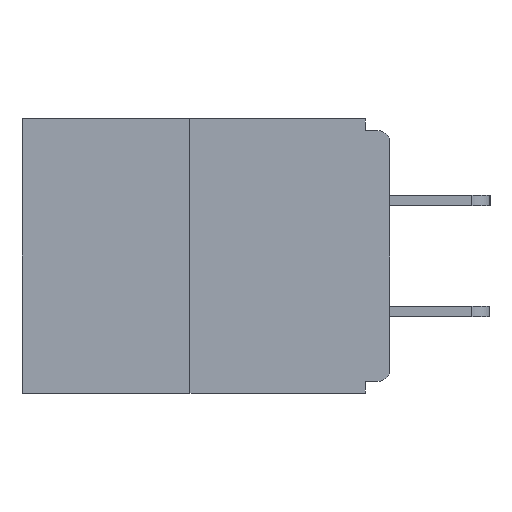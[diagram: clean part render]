
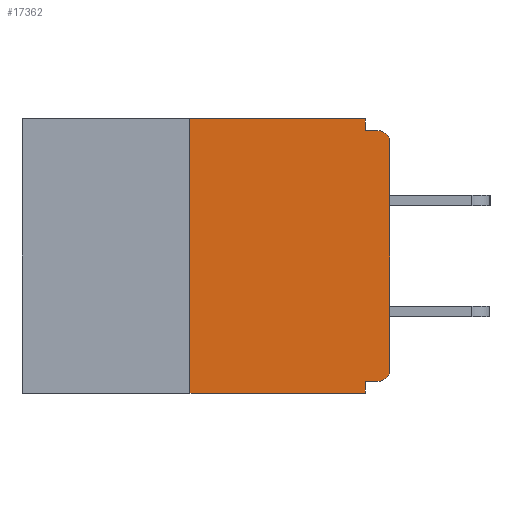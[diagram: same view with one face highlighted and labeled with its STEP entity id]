
A CAD part, left-side view. The second image highlights one B-rep face of the part: STEP entity #17362.
In plain terms, the highlighted planar face has unit normal (-1, 0, 0).
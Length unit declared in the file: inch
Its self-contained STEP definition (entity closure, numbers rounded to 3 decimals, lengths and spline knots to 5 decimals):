
#633 = DIRECTION ( 'NONE',  ( -1., 0., 0. ) ) ;
#658 = LINE ( 'NONE', #7552, #6384 ) ;
#696 = ORIENTED_EDGE ( 'NONE', *, *, #22008, .F. ) ;
#698 = CARTESIAN_POINT ( 'NONE',  ( 0., 0.031, -0.343 ) ) ;
#746 = CARTESIAN_POINT ( 'NONE',  ( 0., 0.031, 0. ) ) ;
#1198 = VECTOR ( 'NONE', #19007, 39.37008 ) ;
#1245 = CIRCLE ( 'NONE', #4268, 0.015 ) ;
#1702 = CARTESIAN_POINT ( 'NONE',  ( 0., 0.46, -0.343 ) ) ;
#2007 = VECTOR ( 'NONE', #16914, 39.37008 ) ;
#2011 = ORIENTED_EDGE ( 'NONE', *, *, #13582, .F. ) ;
#2282 = EDGE_CURVE ( 'NONE', #7714, #10179, #658, .T. ) ;
#2679 = PLANE ( 'NONE',  #21142 ) ;
#2697 = VERTEX_POINT ( 'NONE', #16904 ) ;
#2753 = EDGE_CURVE ( 'NONE', #10179, #21299, #7271, .T. ) ;
#2975 = CARTESIAN_POINT ( 'NONE',  ( 0., 0., -0.313 ) ) ;
#3188 = CARTESIAN_POINT ( 'NONE',  ( 0., 0.25, 0. ) ) ;
#4268 = AXIS2_PLACEMENT_3D ( 'NONE', #5613, #16413, #18456 ) ;
#4496 = LINE ( 'NONE', #698, #1198 ) ;
#4762 = ORIENTED_EDGE ( 'NONE', *, *, #13881, .T. ) ;
#4852 = ORIENTED_EDGE ( 'NONE', *, *, #16057, .F. ) ;
#5162 = CARTESIAN_POINT ( 'NONE',  ( 0., 0., -0.015 ) ) ;
#5386 = LINE ( 'NONE', #5162, #18011 ) ;
#5613 = CARTESIAN_POINT ( 'NONE',  ( 0., 0.015, -0.313 ) ) ;
#5687 = CARTESIAN_POINT ( 'NONE',  ( 0., 0.25, 0. ) ) ;
#5970 = DIRECTION ( 'NONE',  ( 0., 0., -1. ) ) ;
#5994 = EDGE_LOOP ( 'NONE', ( #7019, #18274, #4762, #4852, #2011, #18124, #6277, #15535, #7872, #696 ) ) ;
#6277 = ORIENTED_EDGE ( 'NONE', *, *, #2282, .T. ) ;
#6374 = CARTESIAN_POINT ( 'NONE',  ( 0., 0.015, -0.328 ) ) ;
#6384 = VECTOR ( 'NONE', #18962, 39.37008 ) ;
#6940 = LINE ( 'NONE', #1702, #16783 ) ;
#7019 = ORIENTED_EDGE ( 'NONE', *, *, #7269, .F. ) ;
#7269 = EDGE_CURVE ( 'NONE', #18222, #12796, #14925, .T. ) ;
#7271 = CIRCLE ( 'NONE', #18394, 0.015 ) ;
#7540 = CARTESIAN_POINT ( 'NONE',  ( 0., 0., -0.328 ) ) ;
#7552 = CARTESIAN_POINT ( 'NONE',  ( 0., 0., 0. ) ) ;
#7714 = VERTEX_POINT ( 'NONE', #2975 ) ;
#7872 = ORIENTED_EDGE ( 'NONE', *, *, #20592, .F. ) ;
#8287 = CARTESIAN_POINT ( 'NONE',  ( 0., 0.46, 0. ) ) ;
#8774 = VECTOR ( 'NONE', #14571, 39.37008 ) ;
#9025 = CARTESIAN_POINT ( 'NONE',  ( 0., 0.46, 0. ) ) ;
#9357 = DIRECTION ( 'NONE',  ( 0., -1., 0. ) ) ;
#9393 = EDGE_CURVE ( 'NONE', #10746, #7714, #1245, .T. ) ;
#9884 = VECTOR ( 'NONE', #11315, 39.37008 ) ;
#10179 = VERTEX_POINT ( 'NONE', #17896 ) ;
#10746 = VERTEX_POINT ( 'NONE', #6374 ) ;
#11239 = CARTESIAN_POINT ( 'NONE',  ( 0., 0.031, -0.015 ) ) ;
#11315 = DIRECTION ( 'NONE',  ( 0., 1., 0. ) ) ;
#11369 = DIRECTION ( 'NONE',  ( 0., 0., 1. ) ) ;
#11543 = LINE ( 'NONE', #746, #2007 ) ;
#11707 = DIRECTION ( 'NONE',  ( 1., 0., 0. ) ) ;
#12796 = VERTEX_POINT ( 'NONE', #22966 ) ;
#13266 = VERTEX_POINT ( 'NONE', #19332 ) ;
#13582 = EDGE_CURVE ( 'NONE', #10746, #2697, #16565, .T. ) ;
#13850 = VECTOR ( 'NONE', #11369, 39.37008 ) ;
#13881 = EDGE_CURVE ( 'NONE', #16589, #13266, #6940, .T. ) ;
#14298 = DIRECTION ( 'NONE',  ( 0., -1., 0. ) ) ;
#14571 = DIRECTION ( 'NONE',  ( 0., -1., 0. ) ) ;
#14925 = LINE ( 'NONE', #9025, #8774 ) ;
#15535 = ORIENTED_EDGE ( 'NONE', *, *, #2753, .T. ) ;
#15632 = DIRECTION ( 'NONE',  ( 0., 0., -1. ) ) ;
#16057 = EDGE_CURVE ( 'NONE', #2697, #13266, #4496, .T. ) ;
#16413 = DIRECTION ( 'NONE',  ( -1., 0., 0. ) ) ;
#16565 = LINE ( 'NONE', #7540, #9884 ) ;
#16589 = VERTEX_POINT ( 'NONE', #17599 ) ;
#16783 = VECTOR ( 'NONE', #14298, 39.37008 ) ;
#16847 = EDGE_CURVE ( 'NONE', #16589, #18222, #22118, .T. ) ;
#16904 = CARTESIAN_POINT ( 'NONE',  ( 0., 0.031, -0.328 ) ) ;
#16914 = DIRECTION ( 'NONE',  ( 0., 0., -1. ) ) ;
#17362 = ADVANCED_FACE ( 'NONE', ( #23078 ), #2679, .F. ) ;
#17599 = CARTESIAN_POINT ( 'NONE',  ( 0., 0.25, -0.343 ) ) ;
#17896 = CARTESIAN_POINT ( 'NONE',  ( 0., 0., -0.03 ) ) ;
#18011 = VECTOR ( 'NONE', #9357, 39.37008 ) ;
#18124 = ORIENTED_EDGE ( 'NONE', *, *, #9393, .T. ) ;
#18222 = VERTEX_POINT ( 'NONE', #3188 ) ;
#18274 = ORIENTED_EDGE ( 'NONE', *, *, #16847, .F. ) ;
#18394 = AXIS2_PLACEMENT_3D ( 'NONE', #20250, #633, #5970 ) ;
#18456 = DIRECTION ( 'NONE',  ( 0., 0., -1. ) ) ;
#18935 = VERTEX_POINT ( 'NONE', #11239 ) ;
#18962 = DIRECTION ( 'NONE',  ( 0., 0., 1. ) ) ;
#19007 = DIRECTION ( 'NONE',  ( 0., 0., -1. ) ) ;
#19332 = CARTESIAN_POINT ( 'NONE',  ( 0., 0.031, -0.343 ) ) ;
#20250 = CARTESIAN_POINT ( 'NONE',  ( 0., 0.015, -0.03 ) ) ;
#20592 = EDGE_CURVE ( 'NONE', #18935, #21299, #5386, .T. ) ;
#21142 = AXIS2_PLACEMENT_3D ( 'NONE', #8287, #11707, #15632 ) ;
#21299 = VERTEX_POINT ( 'NONE', #22759 ) ;
#22008 = EDGE_CURVE ( 'NONE', #12796, #18935, #11543, .T. ) ;
#22118 = LINE ( 'NONE', #5687, #13850 ) ;
#22759 = CARTESIAN_POINT ( 'NONE',  ( 0., 0.015, -0.015 ) ) ;
#22966 = CARTESIAN_POINT ( 'NONE',  ( 0., 0.031, 0. ) ) ;
#23078 = FACE_OUTER_BOUND ( 'NONE', #5994, .T. ) ;
